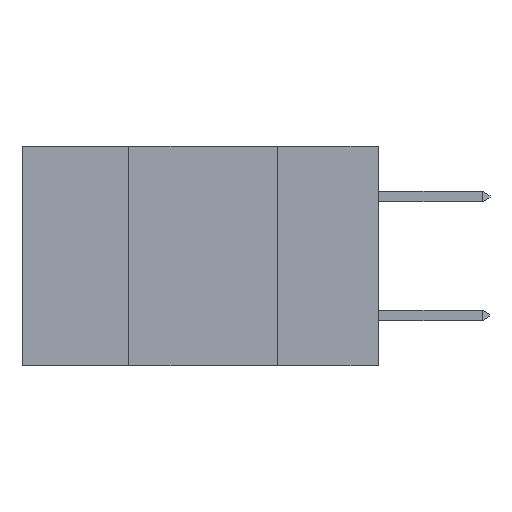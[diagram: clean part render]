
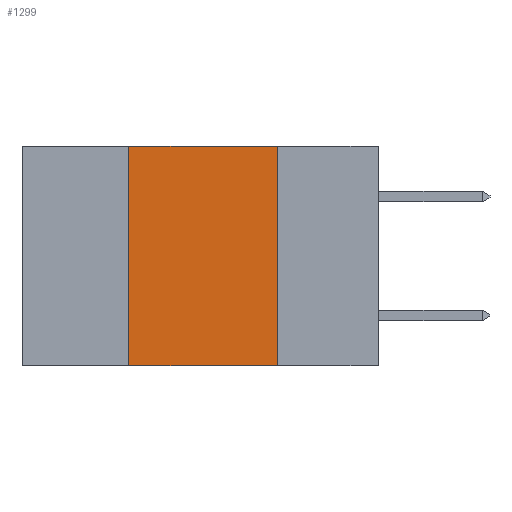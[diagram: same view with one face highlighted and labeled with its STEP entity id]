
A CAD part, left-side view. The second image highlights one B-rep face of the part: STEP entity #1299.
In plain terms, the highlighted planar face has unit normal (-1, 0, 0).
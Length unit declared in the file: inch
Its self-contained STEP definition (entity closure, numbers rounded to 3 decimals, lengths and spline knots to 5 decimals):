
#433 = VECTOR ( 'NONE', #5567, 39.37008 ) ;
#802 = LINE ( 'NONE', #8269, #7421 ) ;
#1099 = AXIS2_PLACEMENT_3D ( 'NONE', #5502, #1393, #4194 ) ;
#1163 = ORIENTED_EDGE ( 'NONE', *, *, #4335, .F. ) ;
#1184 = CARTESIAN_POINT ( 'NONE',  ( 0., 0.42, 0. ) ) ;
#1299 = ADVANCED_FACE ( 'NONE', ( #2348 ), #7867, .F. ) ;
#1393 = DIRECTION ( 'NONE',  ( 1., 0., 0. ) ) ;
#1653 = LINE ( 'NONE', #5559, #3718 ) ;
#2055 = CARTESIAN_POINT ( 'NONE',  ( 0., 0.42, -0.37 ) ) ;
#2348 = FACE_OUTER_BOUND ( 'NONE', #4728, .T. ) ;
#2686 = LINE ( 'NONE', #10046, #9002 ) ;
#3102 = ORIENTED_EDGE ( 'NONE', *, *, #5510, .T. ) ;
#3394 = VERTEX_POINT ( 'NONE', #1184 ) ;
#3718 = VECTOR ( 'NONE', #8683, 39.37008 ) ;
#4194 = DIRECTION ( 'NONE',  ( 0., 0., -1. ) ) ;
#4335 = EDGE_CURVE ( 'NONE', #5822, #3394, #2686, .T. ) ;
#4728 = EDGE_LOOP ( 'NONE', ( #6542, #8972, #1163, #3102 ) ) ;
#5059 = VERTEX_POINT ( 'NONE', #10073 ) ;
#5502 = CARTESIAN_POINT ( 'NONE',  ( 0., 0.6, 0. ) ) ;
#5510 = EDGE_CURVE ( 'NONE', #5822, #5059, #7132, .T. ) ;
#5559 = CARTESIAN_POINT ( 'NONE',  ( 0., 0.6, 0. ) ) ;
#5567 = DIRECTION ( 'NONE',  ( 0., -1., 0. ) ) ;
#5623 = CARTESIAN_POINT ( 'NONE',  ( 0., 0.6, -0.37 ) ) ;
#5822 = VERTEX_POINT ( 'NONE', #2055 ) ;
#6542 = ORIENTED_EDGE ( 'NONE', *, *, #9359, .F. ) ;
#6781 = CARTESIAN_POINT ( 'NONE',  ( 0., 0.17, 0. ) ) ;
#7132 = LINE ( 'NONE', #5623, #433 ) ;
#7421 = VECTOR ( 'NONE', #9030, 39.37008 ) ;
#7564 = VERTEX_POINT ( 'NONE', #6781 ) ;
#7867 = PLANE ( 'NONE',  #1099 ) ;
#8269 = CARTESIAN_POINT ( 'NONE',  ( 0., 0.17, 0. ) ) ;
#8683 = DIRECTION ( 'NONE',  ( 0., -1., 0. ) ) ;
#8972 = ORIENTED_EDGE ( 'NONE', *, *, #9770, .F. ) ;
#9002 = VECTOR ( 'NONE', #10056, 39.37008 ) ;
#9030 = DIRECTION ( 'NONE',  ( 0., 0., -1. ) ) ;
#9359 = EDGE_CURVE ( 'NONE', #7564, #5059, #802, .T. ) ;
#9770 = EDGE_CURVE ( 'NONE', #3394, #7564, #1653, .T. ) ;
#10046 = CARTESIAN_POINT ( 'NONE',  ( 0., 0.42, 0. ) ) ;
#10056 = DIRECTION ( 'NONE',  ( 0., 0., 1. ) ) ;
#10073 = CARTESIAN_POINT ( 'NONE',  ( 0., 0.17, -0.37 ) ) ;
